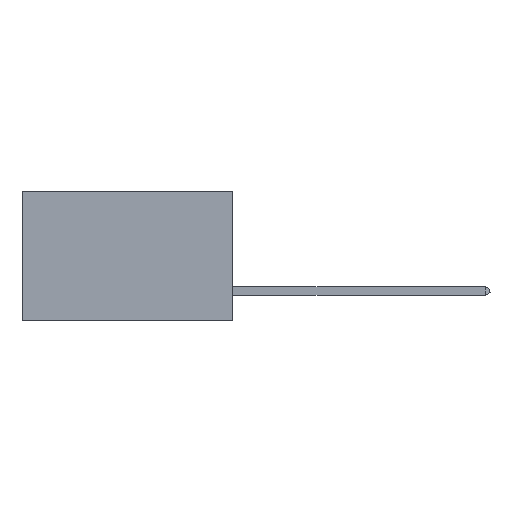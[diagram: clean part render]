
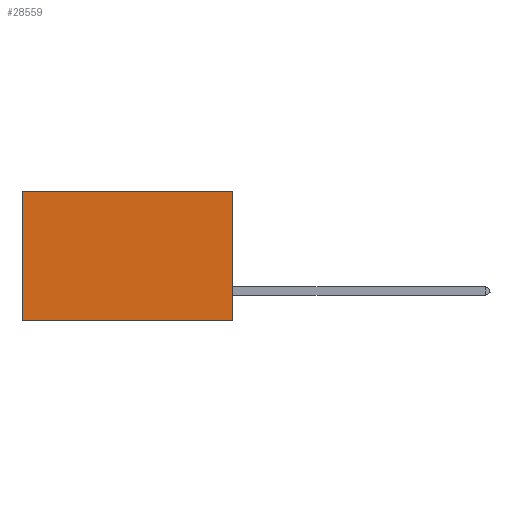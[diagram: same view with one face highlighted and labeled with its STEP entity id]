
A CAD part, left-side view. The second image highlights one B-rep face of the part: STEP entity #28559.
In plain terms, the highlighted planar face has unit normal (-1, 0, 0).
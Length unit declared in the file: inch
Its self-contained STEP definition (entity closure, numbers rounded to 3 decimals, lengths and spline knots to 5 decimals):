
#2961 = FACE_OUTER_BOUND ( 'NONE', #12398, .T. ) ;
#3876 = VECTOR ( 'NONE', #12804, 39.37008 ) ;
#4751 = EDGE_CURVE ( 'NONE', #12242, #17050, #13084, .T. ) ;
#5275 = DIRECTION ( 'NONE',  ( 0., 0., -1. ) ) ;
#5491 = CARTESIAN_POINT ( 'NONE',  ( 0.2875, 0.6, 0. ) ) ;
#8430 = VECTOR ( 'NONE', #17069, 39.37008 ) ;
#8829 = CARTESIAN_POINT ( 'NONE',  ( 0.2875, 0.6, -0.37 ) ) ;
#10464 = DIRECTION ( 'NONE',  ( 1., 0., 0. ) ) ;
#10708 = ORIENTED_EDGE ( 'NONE', *, *, #4751, .F. ) ;
#10927 = VERTEX_POINT ( 'NONE', #5491 ) ;
#11219 = EDGE_CURVE ( 'NONE', #17050, #12641, #16389, .T. ) ;
#12242 = VERTEX_POINT ( 'NONE', #19358 ) ;
#12398 = EDGE_LOOP ( 'NONE', ( #16484, #19717, #10708, #25963 ) ) ;
#12629 = LINE ( 'NONE', #14956, #21098 ) ;
#12641 = VERTEX_POINT ( 'NONE', #8829 ) ;
#12804 = DIRECTION ( 'NONE',  ( 0., 0., -1. ) ) ;
#13084 = LINE ( 'NONE', #22820, #3876 ) ;
#14956 = CARTESIAN_POINT ( 'NONE',  ( 0.2875, 0.6, 0. ) ) ;
#16188 = LINE ( 'NONE', #31777, #8430 ) ;
#16389 = LINE ( 'NONE', #28490, #23266 ) ;
#16484 = ORIENTED_EDGE ( 'NONE', *, *, #28391, .T. ) ;
#17050 = VERTEX_POINT ( 'NONE', #22627 ) ;
#17069 = DIRECTION ( 'NONE',  ( 0., 1., 0. ) ) ;
#18537 = AXIS2_PLACEMENT_3D ( 'NONE', #19901, #10464, #5275 ) ;
#18996 = DIRECTION ( 'NONE',  ( 0., 1., 0. ) ) ;
#19358 = CARTESIAN_POINT ( 'NONE',  ( 0.2875, 0., 0. ) ) ;
#19717 = ORIENTED_EDGE ( 'NONE', *, *, #11219, .F. ) ;
#19901 = CARTESIAN_POINT ( 'NONE',  ( 0.2875, 0., 0. ) ) ;
#21098 = VECTOR ( 'NONE', #31977, 39.37008 ) ;
#22627 = CARTESIAN_POINT ( 'NONE',  ( 0.2875, 0., -0.37 ) ) ;
#22820 = CARTESIAN_POINT ( 'NONE',  ( 0.2875, 0., 0. ) ) ;
#23266 = VECTOR ( 'NONE', #18996, 39.37008 ) ;
#25171 = PLANE ( 'NONE',  #18537 ) ;
#25963 = ORIENTED_EDGE ( 'NONE', *, *, #27303, .T. ) ;
#27303 = EDGE_CURVE ( 'NONE', #12242, #10927, #16188, .T. ) ;
#28391 = EDGE_CURVE ( 'NONE', #10927, #12641, #12629, .T. ) ;
#28490 = CARTESIAN_POINT ( 'NONE',  ( 0.2875, 0., -0.37 ) ) ;
#28559 = ADVANCED_FACE ( 'NONE', ( #2961 ), #25171, .F. ) ;
#31777 = CARTESIAN_POINT ( 'NONE',  ( 0.2875, 0., 0. ) ) ;
#31977 = DIRECTION ( 'NONE',  ( 0., 0., -1. ) ) ;
